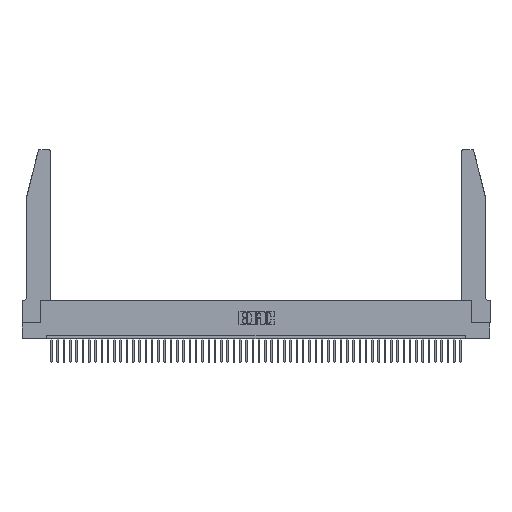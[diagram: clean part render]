
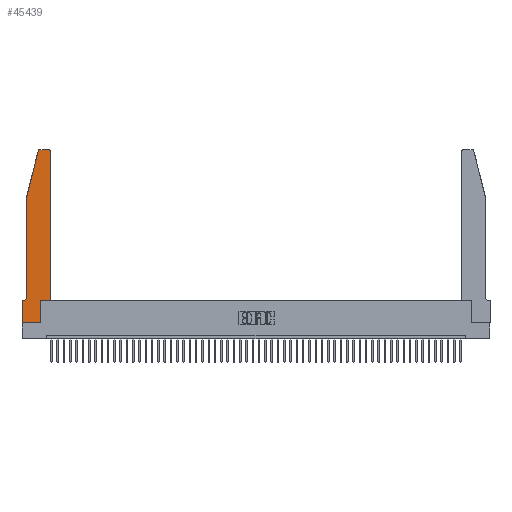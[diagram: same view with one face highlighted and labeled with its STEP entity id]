
A CAD part, top view. The second image highlights one B-rep face of the part: STEP entity #45439.
In plain terms, the highlighted planar face has unit normal (0, 0, 1).
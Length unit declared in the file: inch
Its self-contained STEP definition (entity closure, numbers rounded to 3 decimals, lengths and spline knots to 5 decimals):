
#79 = CARTESIAN_POINT ( 'NONE',  ( 0., 0.35, 0.37 ) ) ;
#191 = VERTEX_POINT ( 'NONE', #39979 ) ;
#368 = DIRECTION ( 'NONE',  ( 1., 0., 0. ) ) ;
#919 = CARTESIAN_POINT ( 'NONE',  ( 0.0755, 2., 0.37 ) ) ;
#1046 = LINE ( 'NONE', #23799, #27048 ) ;
#1160 = VECTOR ( 'NONE', #50556, 39.37008 ) ;
#1755 = VECTOR ( 'NONE', #23444, 39.37008 ) ;
#2453 = LINE ( 'NONE', #30790, #45720 ) ;
#3805 = ORIENTED_EDGE ( 'NONE', *, *, #27708, .T. ) ;
#4271 = EDGE_CURVE ( 'NONE', #20826, #22635, #19057, .T. ) ;
#5146 = EDGE_CURVE ( 'NONE', #13732, #23220, #1046, .T. ) ;
#5456 = CIRCLE ( 'NONE', #14622, 0.03 ) ;
#5948 = VERTEX_POINT ( 'NONE', #7725 ) ;
#6250 = VERTEX_POINT ( 'NONE', #39821 ) ;
#7725 = CARTESIAN_POINT ( 'NONE',  ( 0.284, 2.75, 0.37 ) ) ;
#8697 = CARTESIAN_POINT ( 'NONE',  ( 0.4505, 0.35, 0.37 ) ) ;
#10009 = DIRECTION ( 'NONE',  ( 0., 0., -1. ) ) ;
#10338 = DIRECTION ( 'NONE',  ( 1., 0., 0. ) ) ;
#10500 = VERTEX_POINT ( 'NONE', #11113 ) ;
#10947 = ORIENTED_EDGE ( 'NONE', *, *, #17307, .T. ) ;
#11113 = CARTESIAN_POINT ( 'NONE',  ( 0.0755, 0.42, 0.37 ) ) ;
#11864 = ORIENTED_EDGE ( 'NONE', *, *, #4271, .T. ) ;
#11874 = EDGE_CURVE ( 'NONE', #45544, #191, #5456, .T. ) ;
#12306 = LINE ( 'NONE', #8697, #26599 ) ;
#12973 = LINE ( 'NONE', #19053, #45826 ) ;
#13374 = VERTEX_POINT ( 'NONE', #19573 ) ;
#13469 = CIRCLE ( 'NONE', #16984, 0.07 ) ;
#13732 = VERTEX_POINT ( 'NONE', #15083 ) ;
#14541 = CARTESIAN_POINT ( 'NONE',  ( 0.4205, 2.72, 0.37 ) ) ;
#14586 = DIRECTION ( 'NONE',  ( 1., 0., 0. ) ) ;
#14622 = AXIS2_PLACEMENT_3D ( 'NONE', #14541, #38594, #19006 ) ;
#15083 = CARTESIAN_POINT ( 'NONE',  ( 0., 0., 0.37 ) ) ;
#15279 = CARTESIAN_POINT ( 'NONE',  ( 0.0755, 2., 0.37 ) ) ;
#15344 = ORIENTED_EDGE ( 'NONE', *, *, #47346, .T. ) ;
#16984 = AXIS2_PLACEMENT_3D ( 'NONE', #33843, #10009, #42039 ) ;
#17307 = EDGE_CURVE ( 'NONE', #33653, #13732, #34599, .T. ) ;
#18929 = EDGE_LOOP ( 'NONE', ( #46292, #34687, #11864, #15344, #35798, #3805, #10947, #19589, #33937, #28354, #21011, #38781 ) ) ;
#18981 = DIRECTION ( 'NONE',  ( -1., 0., 0. ) ) ;
#19006 = DIRECTION ( 'NONE',  ( 1., 0., 0. ) ) ;
#19053 = CARTESIAN_POINT ( 'NONE',  ( 0.4505, 0.35, 0.37 ) ) ;
#19057 = LINE ( 'NONE', #42637, #1160 ) ;
#19573 = CARTESIAN_POINT ( 'NONE',  ( 0.0055, 0.35, 0.37 ) ) ;
#19589 = ORIENTED_EDGE ( 'NONE', *, *, #5146, .T. ) ;
#19661 = CARTESIAN_POINT ( 'NONE',  ( 0.2865, 0.35, 0.37 ) ) ;
#20588 = DIRECTION ( 'NONE',  ( 0., 1., 0. ) ) ;
#20826 = VERTEX_POINT ( 'NONE', #50153 ) ;
#20944 = VECTOR ( 'NONE', #25095, 39.37008 ) ;
#21011 = ORIENTED_EDGE ( 'NONE', *, *, #27101, .T. ) ;
#22042 = DIRECTION ( 'NONE',  ( 0., 0., 1. ) ) ;
#22579 = EDGE_CURVE ( 'NONE', #191, #5948, #45032, .T. ) ;
#22635 = VERTEX_POINT ( 'NONE', #15279 ) ;
#23211 = PLANE ( 'NONE',  #49758 ) ;
#23220 = VERTEX_POINT ( 'NONE', #37914 ) ;
#23444 = DIRECTION ( 'NONE',  ( -1., 0., 0. ) ) ;
#23799 = CARTESIAN_POINT ( 'NONE',  ( 0., 0., 0.37 ) ) ;
#24703 = DIRECTION ( 'NONE',  ( 0., -1., 0. ) ) ;
#25095 = DIRECTION ( 'NONE',  ( 0., -1., 0. ) ) ;
#25499 = CARTESIAN_POINT ( 'NONE',  ( 0.284, 2.72, 0.37 ) ) ;
#26599 = VECTOR ( 'NONE', #20588, 39.37008 ) ;
#26641 = CARTESIAN_POINT ( 'NONE',  ( 0., 0., 0.37 ) ) ;
#26950 = CARTESIAN_POINT ( 'NONE',  ( 0.2605, 2.75, 0.37 ) ) ;
#27048 = VECTOR ( 'NONE', #368, 39.37008 ) ;
#27101 = EDGE_CURVE ( 'NONE', #37463, #45544, #12306, .T. ) ;
#27708 = EDGE_CURVE ( 'NONE', #13374, #33653, #2453, .T. ) ;
#28354 = ORIENTED_EDGE ( 'NONE', *, *, #48230, .T. ) ;
#28508 = LINE ( 'NONE', #19661, #50856 ) ;
#30440 = VECTOR ( 'NONE', #24703, 39.37008 ) ;
#30790 = CARTESIAN_POINT ( 'NONE',  ( 0.0755, 0.35, 0.37 ) ) ;
#31189 = DIRECTION ( 'NONE',  ( 1., 0., 0. ) ) ;
#31558 = AXIS2_PLACEMENT_3D ( 'NONE', #25499, #22042, #10338 ) ;
#33537 = CARTESIAN_POINT ( 'NONE',  ( 0.4505, 0.35, 0.37 ) ) ;
#33653 = VERTEX_POINT ( 'NONE', #48249 ) ;
#33843 = CARTESIAN_POINT ( 'NONE',  ( 0.0055, 0.42, 0.37 ) ) ;
#33937 = ORIENTED_EDGE ( 'NONE', *, *, #47780, .T. ) ;
#34599 = LINE ( 'NONE', #26641, #20944 ) ;
#34687 = ORIENTED_EDGE ( 'NONE', *, *, #48493, .T. ) ;
#35268 = DIRECTION ( 'NONE',  ( 0., 1., 0. ) ) ;
#35798 = ORIENTED_EDGE ( 'NONE', *, *, #35956, .T. ) ;
#35956 = EDGE_CURVE ( 'NONE', #10500, #13374, #13469, .T. ) ;
#37463 = VERTEX_POINT ( 'NONE', #33537 ) ;
#37914 = CARTESIAN_POINT ( 'NONE',  ( 0.2865, 0., 0.37 ) ) ;
#38594 = DIRECTION ( 'NONE',  ( 0., 0., 1. ) ) ;
#38781 = ORIENTED_EDGE ( 'NONE', *, *, #11874, .T. ) ;
#39821 = CARTESIAN_POINT ( 'NONE',  ( 0.2865, 0.35, 0.37 ) ) ;
#39979 = CARTESIAN_POINT ( 'NONE',  ( 0.4205, 2.75, 0.37 ) ) ;
#40144 = CARTESIAN_POINT ( 'NONE',  ( 0.4505, 2.72, 0.37 ) ) ;
#42039 = DIRECTION ( 'NONE',  ( -1., 0., 0. ) ) ;
#42637 = CARTESIAN_POINT ( 'NONE',  ( 0.0755, 2., 0.37 ) ) ;
#43435 = LINE ( 'NONE', #919, #30440 ) ;
#45032 = LINE ( 'NONE', #26950, #1755 ) ;
#45439 = ADVANCED_FACE ( 'NONE', ( #49786 ), #23211, .T. ) ;
#45544 = VERTEX_POINT ( 'NONE', #40144 ) ;
#45720 = VECTOR ( 'NONE', #18981, 39.37008 ) ;
#45826 = VECTOR ( 'NONE', #14586, 39.37008 ) ;
#46292 = ORIENTED_EDGE ( 'NONE', *, *, #22579, .T. ) ;
#47346 = EDGE_CURVE ( 'NONE', #22635, #10500, #43435, .T. ) ;
#47780 = EDGE_CURVE ( 'NONE', #23220, #6250, #28508, .T. ) ;
#48230 = EDGE_CURVE ( 'NONE', #6250, #37463, #12973, .T. ) ;
#48249 = CARTESIAN_POINT ( 'NONE',  ( 0., 0.35, 0.37 ) ) ;
#48493 = EDGE_CURVE ( 'NONE', #5948, #20826, #50762, .T. ) ;
#49758 = AXIS2_PLACEMENT_3D ( 'NONE', #79, #50933, #31189 ) ;
#49786 = FACE_OUTER_BOUND ( 'NONE', #18929, .T. ) ;
#50153 = CARTESIAN_POINT ( 'NONE',  ( 0.25487, 2.72718, 0.37 ) ) ;
#50556 = DIRECTION ( 'NONE',  ( -0.239, -0.971, 0. ) ) ;
#50762 = CIRCLE ( 'NONE', #31558, 0.03 ) ;
#50856 = VECTOR ( 'NONE', #35268, 39.37008 ) ;
#50933 = DIRECTION ( 'NONE',  ( 0., 0., 1. ) ) ;
